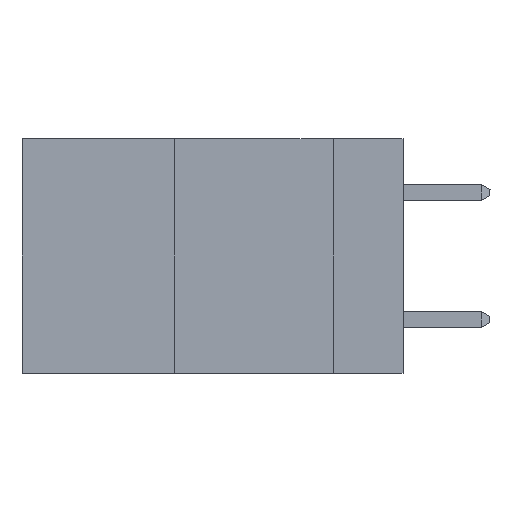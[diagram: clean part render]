
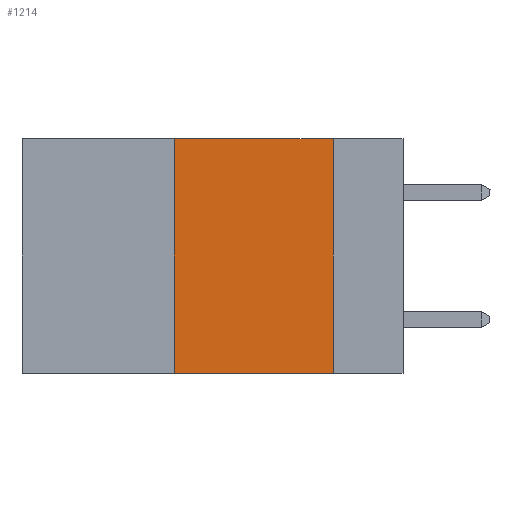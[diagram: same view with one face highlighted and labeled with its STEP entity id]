
A CAD part, left-side view. The second image highlights one B-rep face of the part: STEP entity #1214.
In plain terms, the highlighted planar face has unit normal (-1, 0, 0).
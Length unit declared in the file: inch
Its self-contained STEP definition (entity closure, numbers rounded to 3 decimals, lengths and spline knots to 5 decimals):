
#482 = EDGE_CURVE ( 'NONE', #7964, #7812, #14349, .T. ) ;
#687 = CARTESIAN_POINT ( 'NONE',  ( 0., 0.6, -0.37 ) ) ;
#859 = PLANE ( 'NONE',  #4705 ) ;
#1214 = ADVANCED_FACE ( 'NONE', ( #23808 ), #859, .F. ) ;
#2222 = CARTESIAN_POINT ( 'NONE',  ( 0., 0.36, -0.37 ) ) ;
#2492 = VERTEX_POINT ( 'NONE', #5679 ) ;
#2513 = VECTOR ( 'NONE', #23365, 39.37008 ) ;
#4705 = AXIS2_PLACEMENT_3D ( 'NONE', #18494, #5294, #7482 ) ;
#5294 = DIRECTION ( 'NONE',  ( 1., 0., 0. ) ) ;
#5679 = CARTESIAN_POINT ( 'NONE',  ( 0., 0.11, 0. ) ) ;
#5925 = LINE ( 'NONE', #8021, #2513 ) ;
#7373 = DIRECTION ( 'NONE',  ( 0., -1., 0. ) ) ;
#7482 = DIRECTION ( 'NONE',  ( 0., 0., -1. ) ) ;
#7726 = VECTOR ( 'NONE', #7373, 39.37008 ) ;
#7812 = VERTEX_POINT ( 'NONE', #16853 ) ;
#7964 = VERTEX_POINT ( 'NONE', #2222 ) ;
#8021 = CARTESIAN_POINT ( 'NONE',  ( 0., 0.11, 0. ) ) ;
#8453 = ORIENTED_EDGE ( 'NONE', *, *, #12736, .F. ) ;
#8674 = EDGE_CURVE ( 'NONE', #2492, #7812, #5925, .T. ) ;
#8696 = ORIENTED_EDGE ( 'NONE', *, *, #27438, .F. ) ;
#10676 = DIRECTION ( 'NONE',  ( 0., 0., 1. ) ) ;
#11523 = CARTESIAN_POINT ( 'NONE',  ( 0., 0.6, 0. ) ) ;
#12686 = CARTESIAN_POINT ( 'NONE',  ( 0., 0.36, 0. ) ) ;
#12736 = EDGE_CURVE ( 'NONE', #7964, #20179, #25273, .T. ) ;
#14349 = LINE ( 'NONE', #687, #19560 ) ;
#15550 = CARTESIAN_POINT ( 'NONE',  ( 0., 0.36, 0. ) ) ;
#15990 = DIRECTION ( 'NONE',  ( 0., -1., 0. ) ) ;
#16853 = CARTESIAN_POINT ( 'NONE',  ( 0., 0.11, -0.37 ) ) ;
#17386 = ORIENTED_EDGE ( 'NONE', *, *, #8674, .F. ) ;
#18494 = CARTESIAN_POINT ( 'NONE',  ( 0., 0.6, 0. ) ) ;
#19560 = VECTOR ( 'NONE', #15990, 39.37008 ) ;
#20062 = VECTOR ( 'NONE', #10676, 39.37008 ) ;
#20179 = VERTEX_POINT ( 'NONE', #15550 ) ;
#23365 = DIRECTION ( 'NONE',  ( 0., 0., -1. ) ) ;
#23686 = EDGE_LOOP ( 'NONE', ( #17386, #8696, #8453, #27482 ) ) ;
#23808 = FACE_OUTER_BOUND ( 'NONE', #23686, .T. ) ;
#25273 = LINE ( 'NONE', #12686, #20062 ) ;
#27438 = EDGE_CURVE ( 'NONE', #20179, #2492, #27776, .T. ) ;
#27482 = ORIENTED_EDGE ( 'NONE', *, *, #482, .T. ) ;
#27776 = LINE ( 'NONE', #11523, #7726 ) ;
